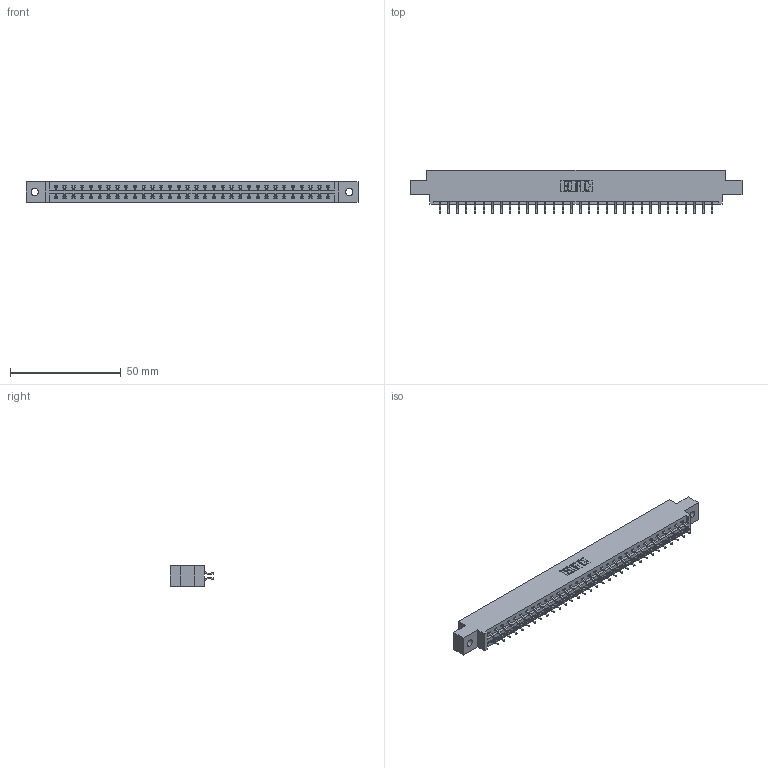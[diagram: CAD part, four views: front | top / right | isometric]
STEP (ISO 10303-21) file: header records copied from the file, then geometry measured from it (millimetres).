
FILE_DESCRIPTION (( 'STEP AP203' ), '1' );
FILE_NAME ('387-064-556-802.STEP', '2018-09-21T08:20:00', ( '' ), ( '' ), 'SwSTEP 2.0', 'SolidWorks 2016', '' );
FILE_SCHEMA (( 'CONFIG_CONTROL_DESIGN' ));
Length unit declared in the file: inch
Products named in the file (3): 337 Part_0.170 Offset - 0.128 Dia; 345-292-001_556 Tail; 387-064-556-802
Assembly tree (65 placements, depth 2):
  387-064-556-802
    337 Part_0.170 Offset - 0.128 Dia
    345-292-001_556 Tail  x64
Bounding box: 149.81 x 19.57 x 9.4 mm (x, y, z)
Volume: 15498.2 mm3; surface area: 17191.3 mm2
Topology: 65 solids, 65 shells, 3958 faces, 11779 edges, 7766 vertices
Faces by surface type: plane 2762, cylinder 1196
Entity records: 26459 total; most frequent: CARTESIAN_POINT 4482, ORIENTED_EDGE 4406, DIRECTION 3819, EDGE_CURVE 2203, VECTOR 2067, LINE 2067, VERTEX_POINT 1466, AXIS2_PLACEMENT_3D 876
